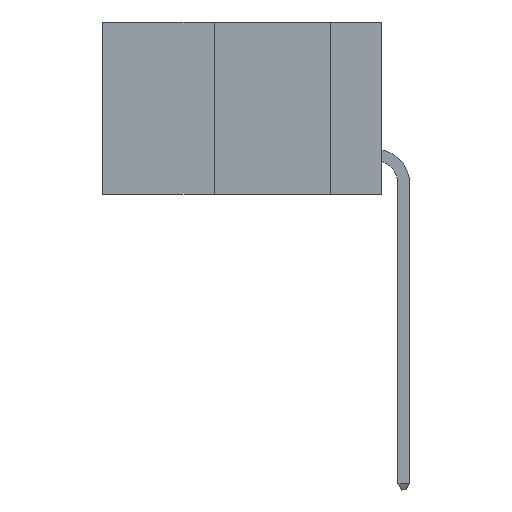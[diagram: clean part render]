
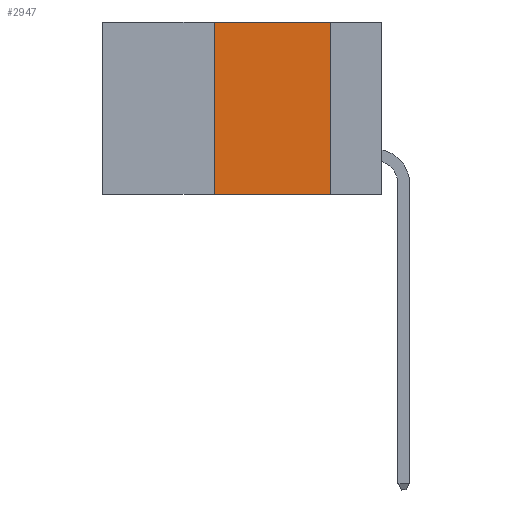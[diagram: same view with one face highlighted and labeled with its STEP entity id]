
A CAD part, left-side view. The second image highlights one B-rep face of the part: STEP entity #2947.
In plain terms, the highlighted planar face has unit normal (-1, 0, 0).
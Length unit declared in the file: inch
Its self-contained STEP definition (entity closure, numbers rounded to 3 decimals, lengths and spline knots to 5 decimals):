
#2947 = ADVANCED_FACE ( 'NONE', ( #38414 ), #41601, .F. ) ;
#4978 = CARTESIAN_POINT ( 'NONE',  ( 0., 0.36, 0. ) ) ;
#7523 = EDGE_CURVE ( 'NONE', #26548, #29611, #9512, .T. ) ;
#8176 = DIRECTION ( 'NONE',  ( 0., 0., -1. ) ) ;
#9078 = VECTOR ( 'NONE', #8176, 39.37008 ) ;
#9176 = ORIENTED_EDGE ( 'NONE', *, *, #18928, .F. ) ;
#9512 = LINE ( 'NONE', #4978, #47683 ) ;
#13739 = DIRECTION ( 'NONE',  ( 0., -1., 0. ) ) ;
#14744 = EDGE_LOOP ( 'NONE', ( #9176, #37018, #26700, #22913 ) ) ;
#16108 = DIRECTION ( 'NONE',  ( 0., 0., 1. ) ) ;
#18884 = LINE ( 'NONE', #23054, #9078 ) ;
#18928 = EDGE_CURVE ( 'NONE', #34303, #44564, #18884, .T. ) ;
#20341 = LINE ( 'NONE', #20852, #22078 ) ;
#20852 = CARTESIAN_POINT ( 'NONE',  ( 0., 0.6, 0. ) ) ;
#22078 = VECTOR ( 'NONE', #13739, 39.37008 ) ;
#22913 = ORIENTED_EDGE ( 'NONE', *, *, #30078, .T. ) ;
#23054 = CARTESIAN_POINT ( 'NONE',  ( 0., 0.11, 0. ) ) ;
#24177 = DIRECTION ( 'NONE',  ( 0., -1., 0. ) ) ;
#26548 = VERTEX_POINT ( 'NONE', #29109 ) ;
#26700 = ORIENTED_EDGE ( 'NONE', *, *, #7523, .F. ) ;
#27265 = AXIS2_PLACEMENT_3D ( 'NONE', #34340, #38186, #44241 ) ;
#29109 = CARTESIAN_POINT ( 'NONE',  ( 0., 0.36, -0.37 ) ) ;
#29611 = VERTEX_POINT ( 'NONE', #46128 ) ;
#30078 = EDGE_CURVE ( 'NONE', #26548, #44564, #45573, .T. ) ;
#34303 = VERTEX_POINT ( 'NONE', #42037 ) ;
#34340 = CARTESIAN_POINT ( 'NONE',  ( 0., 0.6, 0. ) ) ;
#35679 = EDGE_CURVE ( 'NONE', #29611, #34303, #20341, .T. ) ;
#36915 = VECTOR ( 'NONE', #24177, 39.37008 ) ;
#37018 = ORIENTED_EDGE ( 'NONE', *, *, #35679, .F. ) ;
#38186 = DIRECTION ( 'NONE',  ( 1., 0., 0. ) ) ;
#38414 = FACE_OUTER_BOUND ( 'NONE', #14744, .T. ) ;
#41601 = PLANE ( 'NONE',  #27265 ) ;
#41747 = CARTESIAN_POINT ( 'NONE',  ( 0., 0.11, -0.37 ) ) ;
#42037 = CARTESIAN_POINT ( 'NONE',  ( 0., 0.11, 0. ) ) ;
#44241 = DIRECTION ( 'NONE',  ( 0., 0., -1. ) ) ;
#44564 = VERTEX_POINT ( 'NONE', #41747 ) ;
#45573 = LINE ( 'NONE', #46314, #36915 ) ;
#46128 = CARTESIAN_POINT ( 'NONE',  ( 0., 0.36, 0. ) ) ;
#46314 = CARTESIAN_POINT ( 'NONE',  ( 0., 0.6, -0.37 ) ) ;
#47683 = VECTOR ( 'NONE', #16108, 39.37008 ) ;
